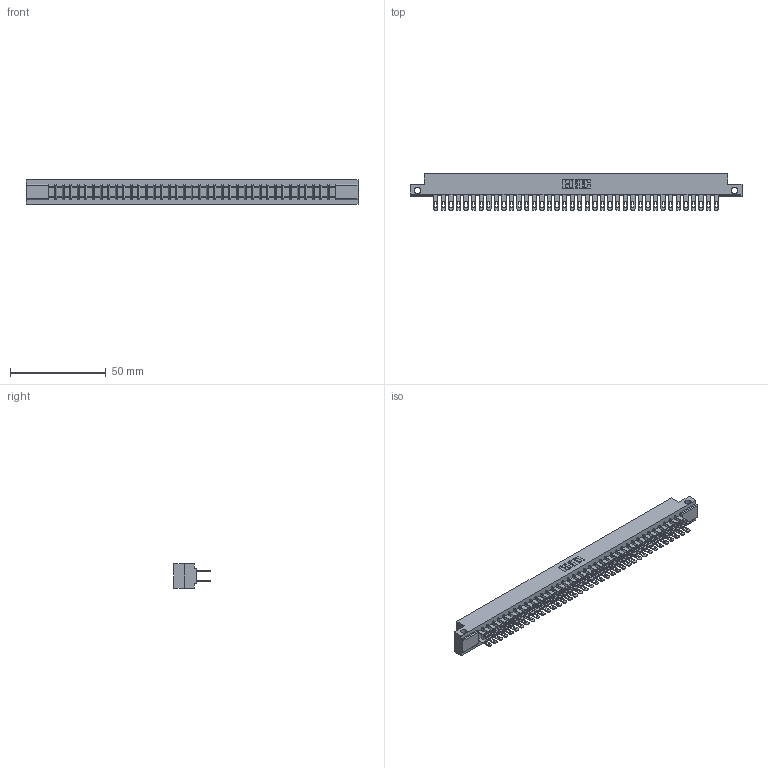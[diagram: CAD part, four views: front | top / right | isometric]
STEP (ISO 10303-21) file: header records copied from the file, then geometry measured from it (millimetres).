
FILE_DESCRIPTION (( 'STEP AP203' ), '1' );
FILE_NAME ('307-076-500-212.STEP', '2019-09-06T21:42:25', ( '' ), ( '' ), 'SwSTEP 2.0', 'SolidWorks 2016', '' );
FILE_SCHEMA (( 'CONFIG_CONTROL_DESIGN' ));
Length unit declared in the file: inch
Products named in the file (3): 307-290-001_500; 307 Part_.128 Dia Side Mounting Holes; 307-076-500-212
Assembly tree (77 placements, depth 2):
  307-076-500-212
    307 Part_.128 Dia Side Mounting Holes
    307-290-001_500  x76
Bounding box: 173.58 x 19.18 x 12.7 mm (x, y, z)
Volume: 18505.9 mm3; surface area: 23757.2 mm2
Topology: 77 solids, 77 shells, 3653 faces, 10203 edges, 6594 vertices
Faces by surface type: plane 2350, cylinder 1225, sphere 78
Entity records: 34262 total; most frequent: CARTESIAN_POINT 5602, ORIENTED_EDGE 5550, DIRECTION 5491, EDGE_CURVE 2775, VECTOR 2125, LINE 2125, VERTEX_POINT 1794, AXIS2_PLACEMENT_3D 1683
